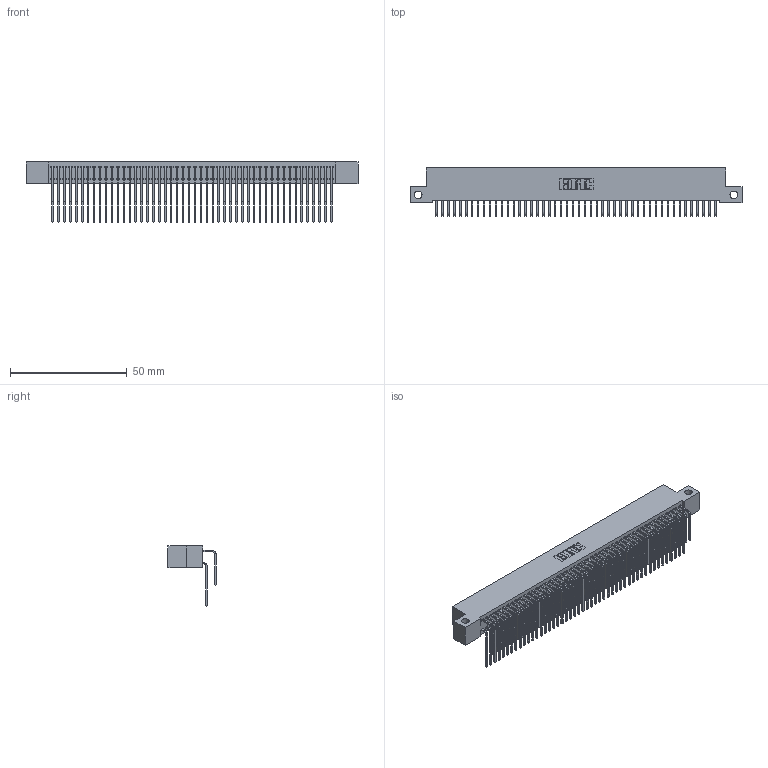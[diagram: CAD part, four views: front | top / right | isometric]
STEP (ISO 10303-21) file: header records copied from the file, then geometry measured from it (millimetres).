
FILE_DESCRIPTION (( 'STEP AP203' ), '1' );
FILE_NAME ('342-096-559-212.STEP', '2019-10-04T16:23:46', ( '' ), ( '' ), 'SwSTEP 2.0', 'SolidWorks 2016', '' );
FILE_SCHEMA (( 'CONFIG_CONTROL_DESIGN' ));
Length unit declared in the file: inch
Products named in the file (4): 342 Part_Side Mount; 345-292-001_558 559 Tail - 1; 345-292-001_559 Tail - 2; 342-096-559-212
Assembly tree (97 placements, depth 2):
  342-096-559-212
    342 Part_Side Mount
    345-292-001_558 559 Tail - 1  x48
    345-292-001_559 Tail - 2  x48
Bounding box: 142.24 x 20.64 x 25.78 mm (x, y, z)
Volume: 13288.5 mm3; surface area: 24123.6 mm2
Topology: 97 solids, 97 shells, 5294 faces, 15755 edges, 10374 vertices
Faces by surface type: plane 3714, cylinder 1580
Entity records: 31759 total; most frequent: CARTESIAN_POINT 5305, ORIENTED_EDGE 5190, DIRECTION 4503, EDGE_CURVE 2595, LINE 2427, VECTOR 2427, VERTEX_POINT 1726, AXIS2_PLACEMENT_3D 1038
